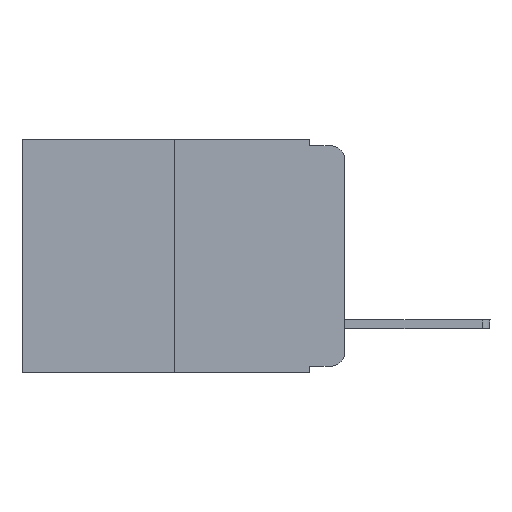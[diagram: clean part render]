
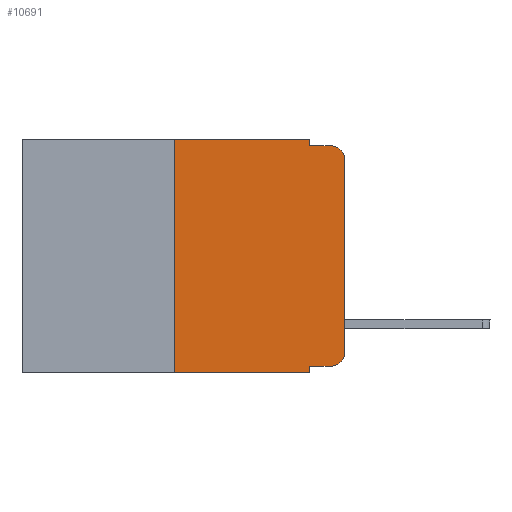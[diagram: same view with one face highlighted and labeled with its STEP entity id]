
A CAD part, left-side view. The second image highlights one B-rep face of the part: STEP entity #10691.
In plain terms, the highlighted planar face has unit normal (-1, 0, 0).
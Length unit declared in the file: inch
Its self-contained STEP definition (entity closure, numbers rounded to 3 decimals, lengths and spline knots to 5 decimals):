
#92 = DIRECTION ( 'NONE',  ( -1., 0., 0. ) ) ;
#441 = CARTESIAN_POINT ( 'NONE',  ( 0., 0., 0. ) ) ;
#565 = CARTESIAN_POINT ( 'NONE',  ( 0., 0.25, 0. ) ) ;
#577 = ORIENTED_EDGE ( 'NONE', *, *, #15258, .T. ) ;
#610 = ORIENTED_EDGE ( 'NONE', *, *, #7130, .F. ) ;
#963 = VERTEX_POINT ( 'NONE', #11905 ) ;
#1076 = EDGE_CURVE ( 'NONE', #7003, #4748, #19405, .T. ) ;
#1141 = ORIENTED_EDGE ( 'NONE', *, *, #8269, .T. ) ;
#1292 = ORIENTED_EDGE ( 'NONE', *, *, #16359, .F. ) ;
#1362 = EDGE_CURVE ( 'NONE', #7003, #963, #6691, .T. ) ;
#1932 = VECTOR ( 'NONE', #17749, 39.37008 ) ;
#2267 = LINE ( 'NONE', #13935, #17146 ) ;
#2593 = FACE_OUTER_BOUND ( 'NONE', #10510, .T. ) ;
#2898 = CARTESIAN_POINT ( 'NONE',  ( 0., 0.473, 0. ) ) ;
#2956 = CIRCLE ( 'NONE', #15151, 0.02 ) ;
#3145 = VECTOR ( 'NONE', #11324, 39.37008 ) ;
#3289 = LINE ( 'NONE', #16978, #6588 ) ;
#4700 = CARTESIAN_POINT ( 'NONE',  ( 0., 0.051, -0.343 ) ) ;
#4748 = VERTEX_POINT ( 'NONE', #4700 ) ;
#4854 = VECTOR ( 'NONE', #6419, 39.37008 ) ;
#5307 = EDGE_CURVE ( 'NONE', #18092, #9403, #17697, .T. ) ;
#5618 = LINE ( 'NONE', #7760, #16481 ) ;
#5638 = CARTESIAN_POINT ( 'NONE',  ( 0., 0.051, -0.01 ) ) ;
#6419 = DIRECTION ( 'NONE',  ( 0., 0., 1. ) ) ;
#6559 = EDGE_CURVE ( 'NONE', #8328, #18092, #7949, .T. ) ;
#6588 = VECTOR ( 'NONE', #12563, 39.37008 ) ;
#6667 = LINE ( 'NONE', #8530, #1932 ) ;
#6691 = LINE ( 'NONE', #14346, #3145 ) ;
#7003 = VERTEX_POINT ( 'NONE', #10838 ) ;
#7130 = EDGE_CURVE ( 'NONE', #13359, #9403, #2267, .T. ) ;
#7360 = ORIENTED_EDGE ( 'NONE', *, *, #7934, .F. ) ;
#7420 = ORIENTED_EDGE ( 'NONE', *, *, #1362, .T. ) ;
#7760 = CARTESIAN_POINT ( 'NONE',  ( 0., 0.051, 0. ) ) ;
#7934 = EDGE_CURVE ( 'NONE', #16470, #17884, #8870, .T. ) ;
#7949 = LINE ( 'NONE', #441, #4854 ) ;
#8208 = ORIENTED_EDGE ( 'NONE', *, *, #9740, .F. ) ;
#8269 = EDGE_CURVE ( 'NONE', #963, #8328, #2956, .T. ) ;
#8328 = VERTEX_POINT ( 'NONE', #12430 ) ;
#8530 = CARTESIAN_POINT ( 'NONE',  ( 0., 0.25, 0. ) ) ;
#8628 = DIRECTION ( 'NONE',  ( 1., 0., 0. ) ) ;
#8694 = DIRECTION ( 'NONE',  ( 0., 0., -1. ) ) ;
#8870 = LINE ( 'NONE', #2898, #18536 ) ;
#9247 = CARTESIAN_POINT ( 'NONE',  ( 0., 0.02, -0.01 ) ) ;
#9266 = DIRECTION ( 'NONE',  ( 0., 0., -1. ) ) ;
#9403 = VERTEX_POINT ( 'NONE', #9247 ) ;
#9450 = DIRECTION ( 'NONE',  ( 0., -1., 0. ) ) ;
#9593 = CARTESIAN_POINT ( 'NONE',  ( 0., 0., -0.03 ) ) ;
#9740 = EDGE_CURVE ( 'NONE', #19028, #16470, #6667, .T. ) ;
#10510 = EDGE_LOOP ( 'NONE', ( #14820, #19042, #610, #1292, #7360, #8208, #577, #19216, #7420, #1141 ) ) ;
#10691 = ADVANCED_FACE ( 'NONE', ( #2593 ), #16172, .F. ) ;
#10838 = CARTESIAN_POINT ( 'NONE',  ( 0., 0.051, -0.333 ) ) ;
#11162 = DIRECTION ( 'NONE',  ( 0., 0., -1. ) ) ;
#11324 = DIRECTION ( 'NONE',  ( 0., -1., 0. ) ) ;
#11418 = CARTESIAN_POINT ( 'NONE',  ( 0., 0.473, 0. ) ) ;
#11905 = CARTESIAN_POINT ( 'NONE',  ( 0., 0.02, -0.333 ) ) ;
#12366 = VECTOR ( 'NONE', #11162, 39.37008 ) ;
#12430 = CARTESIAN_POINT ( 'NONE',  ( 0., 0., -0.313 ) ) ;
#12563 = DIRECTION ( 'NONE',  ( 0., -1., 0. ) ) ;
#12623 = AXIS2_PLACEMENT_3D ( 'NONE', #11418, #8628, #8694 ) ;
#13189 = DIRECTION ( 'NONE',  ( 0., 0., -1. ) ) ;
#13359 = VERTEX_POINT ( 'NONE', #5638 ) ;
#13628 = DIRECTION ( 'NONE',  ( 0., 0., -1. ) ) ;
#13935 = CARTESIAN_POINT ( 'NONE',  ( 0., 0.051, -0.01 ) ) ;
#14346 = CARTESIAN_POINT ( 'NONE',  ( 0., 0.051, -0.333 ) ) ;
#14820 = ORIENTED_EDGE ( 'NONE', *, *, #6559, .T. ) ;
#15151 = AXIS2_PLACEMENT_3D ( 'NONE', #18950, #19021, #13189 ) ;
#15258 = EDGE_CURVE ( 'NONE', #19028, #4748, #3289, .T. ) ;
#16172 = PLANE ( 'NONE',  #12623 ) ;
#16359 = EDGE_CURVE ( 'NONE', #17884, #13359, #5618, .T. ) ;
#16470 = VERTEX_POINT ( 'NONE', #565 ) ;
#16481 = VECTOR ( 'NONE', #9266, 39.37008 ) ;
#16713 = CARTESIAN_POINT ( 'NONE',  ( 0., 0.02, -0.03 ) ) ;
#16862 = AXIS2_PLACEMENT_3D ( 'NONE', #16713, #92, #13628 ) ;
#16978 = CARTESIAN_POINT ( 'NONE',  ( 0., 0.473, -0.343 ) ) ;
#17146 = VECTOR ( 'NONE', #9450, 39.37008 ) ;
#17165 = CARTESIAN_POINT ( 'NONE',  ( 0., 0.051, 0. ) ) ;
#17697 = CIRCLE ( 'NONE', #16862, 0.02 ) ;
#17749 = DIRECTION ( 'NONE',  ( 0., 0., 1. ) ) ;
#17884 = VERTEX_POINT ( 'NONE', #19462 ) ;
#18092 = VERTEX_POINT ( 'NONE', #9593 ) ;
#18436 = CARTESIAN_POINT ( 'NONE',  ( 0., 0.25, -0.343 ) ) ;
#18536 = VECTOR ( 'NONE', #19154, 39.37008 ) ;
#18950 = CARTESIAN_POINT ( 'NONE',  ( 0., 0.02, -0.313 ) ) ;
#19021 = DIRECTION ( 'NONE',  ( -1., 0., 0. ) ) ;
#19028 = VERTEX_POINT ( 'NONE', #18436 ) ;
#19042 = ORIENTED_EDGE ( 'NONE', *, *, #5307, .T. ) ;
#19154 = DIRECTION ( 'NONE',  ( 0., -1., 0. ) ) ;
#19216 = ORIENTED_EDGE ( 'NONE', *, *, #1076, .F. ) ;
#19405 = LINE ( 'NONE', #17165, #12366 ) ;
#19462 = CARTESIAN_POINT ( 'NONE',  ( 0., 0.051, 0. ) ) ;
